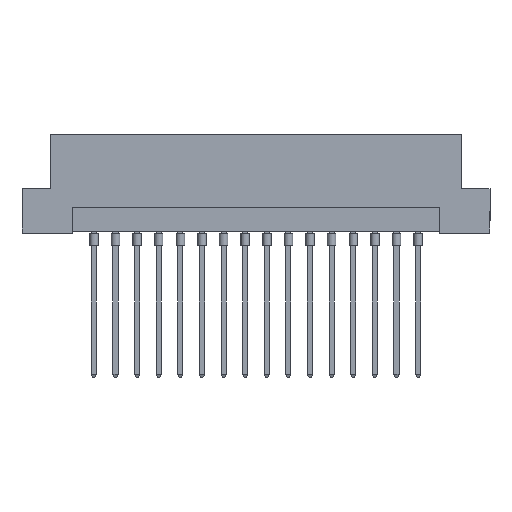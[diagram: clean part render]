
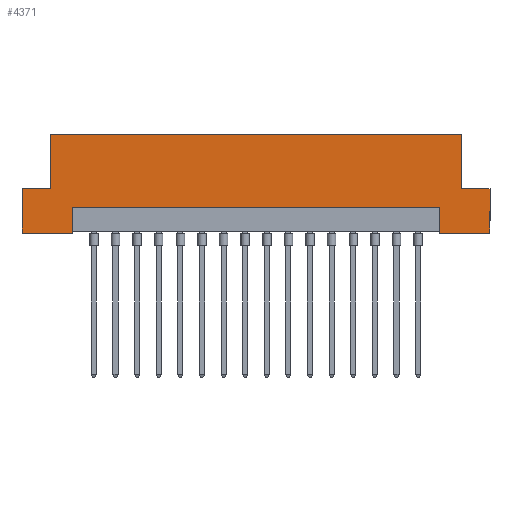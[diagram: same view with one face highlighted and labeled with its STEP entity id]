
A CAD part, front view. The second image highlights one B-rep face of the part: STEP entity #4371.
In plain terms, the highlighted planar face has unit normal (0, -1, 0).
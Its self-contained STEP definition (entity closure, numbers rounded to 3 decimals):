
#89 = VERTEX_POINT ( 'NONE', #6130 ) ;
#104 = CARTESIAN_POINT ( 'NONE',  ( -27.5, -4.3, 0. ) ) ;
#141 = CARTESIAN_POINT ( 'NONE',  ( -21.6, -4.3, 3. ) ) ;
#241 = VERTEX_POINT ( 'NONE', #6912 ) ;
#322 = CARTESIAN_POINT ( 'NONE',  ( 21.6, -4.3, 0. ) ) ;
#350 = CARTESIAN_POINT ( 'NONE',  ( -24.2, -4.3, 5.2 ) ) ;
#372 = CARTESIAN_POINT ( 'NONE',  ( 27.5, -4.3, 0. ) ) ;
#374 = LINE ( 'NONE', #3378, #3587 ) ;
#445 = DIRECTION ( 'NONE',  ( 0., 0., 1. ) ) ;
#593 = LINE ( 'NONE', #4181, #1678 ) ;
#718 = LINE ( 'NONE', #5493, #6292 ) ;
#846 = CARTESIAN_POINT ( 'NONE',  ( -24.2, -4.3, 11.6 ) ) ;
#888 = DIRECTION ( 'NONE',  ( 0., 0., 1. ) ) ;
#961 = DIRECTION ( 'NONE',  ( 0., 0., -1. ) ) ;
#1022 = DIRECTION ( 'NONE',  ( 1., 0., 0. ) ) ;
#1082 = EDGE_CURVE ( 'NONE', #3878, #2945, #718, .T. ) ;
#1101 = DIRECTION ( 'NONE',  ( 0., 0., -1. ) ) ;
#1132 = CARTESIAN_POINT ( 'NONE',  ( 27.5, -4.3, 11.6 ) ) ;
#1136 = CARTESIAN_POINT ( 'NONE',  ( -21.6, -4.3, 0.2 ) ) ;
#1228 = EDGE_CURVE ( 'NONE', #5386, #241, #1617, .T. ) ;
#1282 = ORIENTED_EDGE ( 'NONE', *, *, #2122, .F. ) ;
#1315 = CARTESIAN_POINT ( 'NONE',  ( -27.5, -4.3, 11.6 ) ) ;
#1326 = CARTESIAN_POINT ( 'NONE',  ( 21.6, -4.3, 3. ) ) ;
#1556 = AXIS2_PLACEMENT_3D ( 'NONE', #1132, #3524, #5910 ) ;
#1573 = DIRECTION ( 'NONE',  ( 0., 0., 1. ) ) ;
#1599 = LINE ( 'NONE', #6836, #4584 ) ;
#1617 = LINE ( 'NONE', #372, #7655 ) ;
#1678 = VECTOR ( 'NONE', #7094, 1000. ) ;
#1708 = ORIENTED_EDGE ( 'NONE', *, *, #6699, .T. ) ;
#1806 = ORIENTED_EDGE ( 'NONE', *, *, #7021, .F. ) ;
#1828 = CARTESIAN_POINT ( 'NONE',  ( 27.5, -4.3, 11.6 ) ) ;
#1830 = ORIENTED_EDGE ( 'NONE', *, *, #6449, .T. ) ;
#2122 = EDGE_CURVE ( 'NONE', #89, #2592, #6517, .T. ) ;
#2146 = VECTOR ( 'NONE', #3035, 1000. ) ;
#2177 = EDGE_CURVE ( 'NONE', #4010, #3676, #374, .T. ) ;
#2372 = CARTESIAN_POINT ( 'NONE',  ( -21.6, -4.3, 3. ) ) ;
#2374 = VECTOR ( 'NONE', #961, 1000. ) ;
#2530 = CARTESIAN_POINT ( 'NONE',  ( 27.5, -4.3, 11.6 ) ) ;
#2592 = VERTEX_POINT ( 'NONE', #350 ) ;
#2644 = EDGE_CURVE ( 'NONE', #2592, #6390, #1599, .T. ) ;
#2925 = CARTESIAN_POINT ( 'NONE',  ( -27.5, -4.3, 5.2 ) ) ;
#2945 = VERTEX_POINT ( 'NONE', #7227 ) ;
#3035 = DIRECTION ( 'NONE',  ( 1., 0., 0. ) ) ;
#3056 = PLANE ( 'NONE',  #1556 ) ;
#3203 = VECTOR ( 'NONE', #1573, 1000. ) ;
#3378 = CARTESIAN_POINT ( 'NONE',  ( 24.2, -4.3, 5.2 ) ) ;
#3430 = VERTEX_POINT ( 'NONE', #5604 ) ;
#3524 = DIRECTION ( 'NONE',  ( 0., 1., 0. ) ) ;
#3544 = LINE ( 'NONE', #2372, #2146 ) ;
#3587 = VECTOR ( 'NONE', #445, 1000. ) ;
#3676 = VERTEX_POINT ( 'NONE', #5211 ) ;
#3743 = VECTOR ( 'NONE', #6126, 1000. ) ;
#3799 = VERTEX_POINT ( 'NONE', #141 ) ;
#3876 = CARTESIAN_POINT ( 'NONE',  ( 24.2, -4.3, 5.2 ) ) ;
#3878 = VERTEX_POINT ( 'NONE', #104 ) ;
#4010 = VERTEX_POINT ( 'NONE', #3876 ) ;
#4181 = CARTESIAN_POINT ( 'NONE',  ( 27.5, -4.3, 5.2 ) ) ;
#4220 = LINE ( 'NONE', #1136, #7300 ) ;
#4276 = LINE ( 'NONE', #1315, #2374 ) ;
#4308 = ORIENTED_EDGE ( 'NONE', *, *, #1228, .T. ) ;
#4371 = ADVANCED_FACE ( 'NONE', ( #7198 ), #3056, .F. ) ;
#4528 = LINE ( 'NONE', #6421, #3203 ) ;
#4584 = VECTOR ( 'NONE', #888, 1000. ) ;
#4806 = EDGE_CURVE ( 'NONE', #6390, #3676, #6120, .T. ) ;
#4822 = VECTOR ( 'NONE', #5297, 1000. ) ;
#4857 = ORIENTED_EDGE ( 'NONE', *, *, #1082, .T. ) ;
#4934 = DIRECTION ( 'NONE',  ( 1., 0., 0. ) ) ;
#5021 = LINE ( 'NONE', #2530, #3743 ) ;
#5024 = ORIENTED_EDGE ( 'NONE', *, *, #2177, .T. ) ;
#5211 = CARTESIAN_POINT ( 'NONE',  ( 24.2, -4.3, 11.6 ) ) ;
#5297 = DIRECTION ( 'NONE',  ( 1., 0., 0. ) ) ;
#5386 = VERTEX_POINT ( 'NONE', #322 ) ;
#5493 = CARTESIAN_POINT ( 'NONE',  ( 27.5, -4.3, 0. ) ) ;
#5571 = EDGE_CURVE ( 'NONE', #5386, #5730, #4528, .T. ) ;
#5604 = CARTESIAN_POINT ( 'NONE',  ( 27.5, -4.3, 5.2 ) ) ;
#5730 = VERTEX_POINT ( 'NONE', #1326 ) ;
#5896 = ORIENTED_EDGE ( 'NONE', *, *, #4806, .F. ) ;
#5910 = DIRECTION ( 'NONE',  ( -1., 0., 0. ) ) ;
#6020 = ORIENTED_EDGE ( 'NONE', *, *, #2644, .F. ) ;
#6063 = VECTOR ( 'NONE', #4934, 1000. ) ;
#6092 = ORIENTED_EDGE ( 'NONE', *, *, #7081, .F. ) ;
#6120 = LINE ( 'NONE', #1828, #6063 ) ;
#6126 = DIRECTION ( 'NONE',  ( 0., 0., -1. ) ) ;
#6130 = CARTESIAN_POINT ( 'NONE',  ( -27.5, -4.3, 5.2 ) ) ;
#6230 = ORIENTED_EDGE ( 'NONE', *, *, #6307, .F. ) ;
#6292 = VECTOR ( 'NONE', #6712, 1000. ) ;
#6307 = EDGE_CURVE ( 'NONE', #3430, #241, #5021, .T. ) ;
#6390 = VERTEX_POINT ( 'NONE', #846 ) ;
#6421 = CARTESIAN_POINT ( 'NONE',  ( 21.6, -4.3, 0.2 ) ) ;
#6449 = EDGE_CURVE ( 'NONE', #89, #3878, #4276, .T. ) ;
#6517 = LINE ( 'NONE', #2925, #4822 ) ;
#6699 = EDGE_CURVE ( 'NONE', #3799, #5730, #3544, .T. ) ;
#6712 = DIRECTION ( 'NONE',  ( 1., 0., 0. ) ) ;
#6836 = CARTESIAN_POINT ( 'NONE',  ( -24.2, -4.3, 5.2 ) ) ;
#6912 = CARTESIAN_POINT ( 'NONE',  ( 27.5, -4.3, 0. ) ) ;
#7021 = EDGE_CURVE ( 'NONE', #3799, #2945, #4220, .T. ) ;
#7081 = EDGE_CURVE ( 'NONE', #4010, #3430, #593, .T. ) ;
#7094 = DIRECTION ( 'NONE',  ( 1., 0., 0. ) ) ;
#7198 = FACE_OUTER_BOUND ( 'NONE', #7446, .T. ) ;
#7227 = CARTESIAN_POINT ( 'NONE',  ( -21.6, -4.3, 0. ) ) ;
#7300 = VECTOR ( 'NONE', #1101, 1000. ) ;
#7392 = ORIENTED_EDGE ( 'NONE', *, *, #5571, .F. ) ;
#7446 = EDGE_LOOP ( 'NONE', ( #1708, #7392, #4308, #6230, #6092, #5024, #5896, #6020, #1282, #1830, #4857, #1806 ) ) ;
#7655 = VECTOR ( 'NONE', #1022, 1000. ) ;
